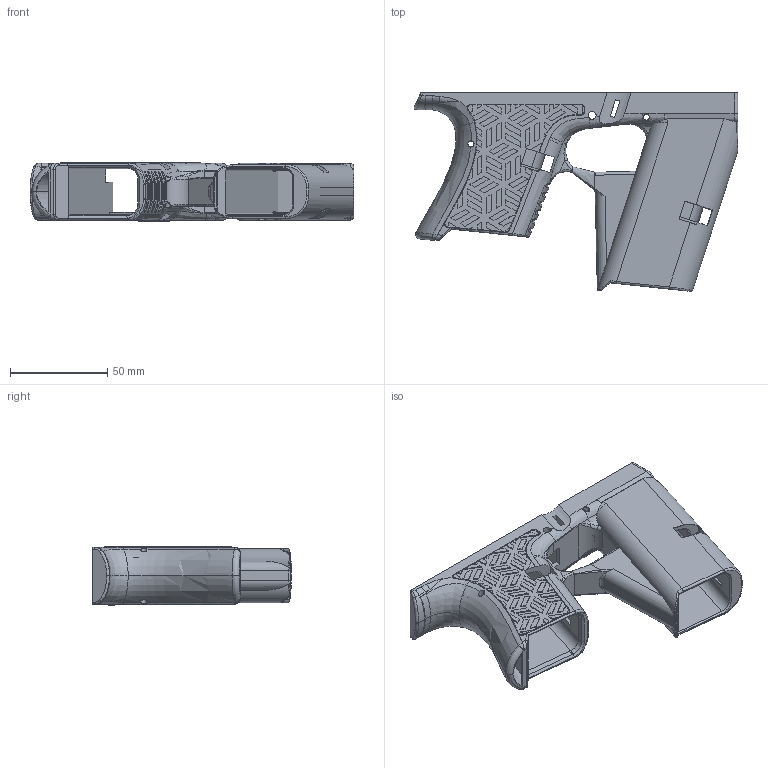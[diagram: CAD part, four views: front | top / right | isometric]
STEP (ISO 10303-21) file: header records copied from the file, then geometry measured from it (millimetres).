
FILE_DESCRIPTION(/* description */ (''),/* implementation_level */ '2;1');
FILE_NAME(/* name */ 'G26 NAO.step',/* time_stamp */ '2022-03-03T12:20:29-07:00',/* author */ (''),/* organization */ (''),/* preprocessor_version */ 'ST-DEVELOPER v18.1',/* originating_system */ 'Autodesk Translation Framework v10.13.0.1454',/* authorisation */ '');
FILE_SCHEMA (('AUTOMOTIVE_DESIGN { 1 0 10303 214 3 1 1 }'));
Products named in the file (1): G26 PDW
Bounding box: 166.88 x 102.34 x 29.99 mm (x, y, z)
Volume: 109401.8 mm3; surface area: 62661.7 mm2
Topology: 1 solids, 1 shells, 1753 faces, 4752 edges, 3029 vertices
Faces by surface type: plane 793, bspline 699, cylinder 206, torus 51, sphere 4
Full cylindrical faces by diameter (mm): 1.903 x1, 3.05 x2, 3.15 x2, 4.111 x2
Entity records: 84642 total; most frequent: CARTESIAN_POINT 46078, ORIENTED_EDGE 9470, DIRECTION 6028, EDGE_CURVE 4735, VERTEX_POINT 3029, LINE 2666, VECTOR 2666, EDGE_LOOP 1830
